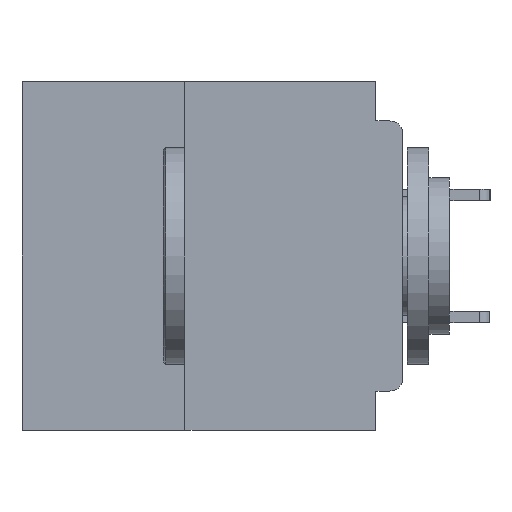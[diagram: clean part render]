
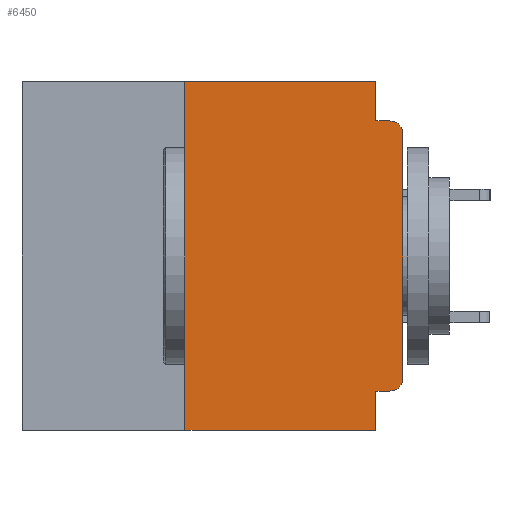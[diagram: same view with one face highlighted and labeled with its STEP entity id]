
A CAD part, left-side view. The second image highlights one B-rep face of the part: STEP entity #6450.
In plain terms, the highlighted planar face has unit normal (-1, 0, 0).
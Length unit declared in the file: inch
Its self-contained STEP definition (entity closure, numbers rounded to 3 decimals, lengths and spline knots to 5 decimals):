
#1854 = CARTESIAN_POINT ( 'NONE',  ( 0., 0.015, -0.34 ) ) ;
#1905 = LINE ( 'NONE', #18883, #39737 ) ;
#2397 = FACE_OUTER_BOUND ( 'NONE', #31106, .T. ) ;
#2887 = ORIENTED_EDGE ( 'NONE', *, *, #15777, .F. ) ;
#3714 = VERTEX_POINT ( 'NONE', #14060 ) ;
#4021 = CARTESIAN_POINT ( 'NONE',  ( 0., 0.25, -0.4 ) ) ;
#4457 = CARTESIAN_POINT ( 'NONE',  ( 0., 0., -0.34 ) ) ;
#5015 = CIRCLE ( 'NONE', #9411, 0.015 ) ;
#5131 = VERTEX_POINT ( 'NONE', #30509 ) ;
#5502 = EDGE_CURVE ( 'NONE', #15753, #28027, #8300, .T. ) ;
#5576 = DIRECTION ( 'NONE',  ( 0., 0., -1. ) ) ;
#5643 = ORIENTED_EDGE ( 'NONE', *, *, #18482, .F. ) ;
#5706 = DIRECTION ( 'NONE',  ( 0., -1., 0. ) ) ;
#5788 = CARTESIAN_POINT ( 'NONE',  ( 0., 0., 0. ) ) ;
#6450 = ADVANCED_FACE ( 'NONE', ( #2397 ), #8949, .F. ) ;
#6662 = DIRECTION ( 'NONE',  ( 0., -1., 0. ) ) ;
#6759 = CARTESIAN_POINT ( 'NONE',  ( 0., 0.031, -0.4 ) ) ;
#7590 = CARTESIAN_POINT ( 'NONE',  ( 0., 0.015, -0.06 ) ) ;
#8300 = LINE ( 'NONE', #6759, #27732 ) ;
#8949 = PLANE ( 'NONE',  #45016 ) ;
#9411 = AXIS2_PLACEMENT_3D ( 'NONE', #7590, #33226, #11280 ) ;
#10138 = LINE ( 'NONE', #44136, #16456 ) ;
#11251 = CARTESIAN_POINT ( 'NONE',  ( 0., 0.031, -0.355 ) ) ;
#11280 = DIRECTION ( 'NONE',  ( 0., 0., -1. ) ) ;
#13911 = LINE ( 'NONE', #4021, #22541 ) ;
#14024 = CARTESIAN_POINT ( 'NONE',  ( 0., 0.25, 0. ) ) ;
#14060 = CARTESIAN_POINT ( 'NONE',  ( 0., 0.015, -0.355 ) ) ;
#14962 = DIRECTION ( 'NONE',  ( 0., 0., 1. ) ) ;
#15753 = VERTEX_POINT ( 'NONE', #11251 ) ;
#15777 = EDGE_CURVE ( 'NONE', #5131, #25336, #13911, .T. ) ;
#16331 = DIRECTION ( 'NONE',  ( 0., 0., -1. ) ) ;
#16456 = VECTOR ( 'NONE', #18564, 39.37008 ) ;
#17638 = ORIENTED_EDGE ( 'NONE', *, *, #32061, .T. ) ;
#18025 = DIRECTION ( 'NONE',  ( 0., 0., -1. ) ) ;
#18482 = EDGE_CURVE ( 'NONE', #24933, #34365, #29122, .T. ) ;
#18564 = DIRECTION ( 'NONE',  ( 0., 1., 0. ) ) ;
#18883 = CARTESIAN_POINT ( 'NONE',  ( 0., 0.031, 0. ) ) ;
#19462 = VECTOR ( 'NONE', #6662, 39.37008 ) ;
#19937 = CARTESIAN_POINT ( 'NONE',  ( 0., 0.031, 0. ) ) ;
#20903 = VERTEX_POINT ( 'NONE', #39258 ) ;
#21000 = EDGE_CURVE ( 'NONE', #25336, #40945, #44535, .T. ) ;
#21565 = CARTESIAN_POINT ( 'NONE',  ( 0., 0.437, 0. ) ) ;
#22482 = ORIENTED_EDGE ( 'NONE', *, *, #45029, .T. ) ;
#22541 = VECTOR ( 'NONE', #14962, 39.37008 ) ;
#22747 = CARTESIAN_POINT ( 'NONE',  ( 0., 0.031, -0.045 ) ) ;
#23201 = ORIENTED_EDGE ( 'NONE', *, *, #30755, .T. ) ;
#24047 = AXIS2_PLACEMENT_3D ( 'NONE', #1854, #27508, #5576 ) ;
#24933 = VERTEX_POINT ( 'NONE', #22747 ) ;
#25336 = VERTEX_POINT ( 'NONE', #14024 ) ;
#25486 = EDGE_CURVE ( 'NONE', #20903, #34365, #5015, .T. ) ;
#26110 = VECTOR ( 'NONE', #5706, 39.37008 ) ;
#26769 = EDGE_CURVE ( 'NONE', #3714, #15753, #10138, .T. ) ;
#27401 = ORIENTED_EDGE ( 'NONE', *, *, #21000, .F. ) ;
#27508 = DIRECTION ( 'NONE',  ( -1., 0., 0. ) ) ;
#27618 = CARTESIAN_POINT ( 'NONE',  ( 0., 0.437, -0.4 ) ) ;
#27732 = VECTOR ( 'NONE', #18025, 39.37008 ) ;
#28027 = VERTEX_POINT ( 'NONE', #36148 ) ;
#28191 = EDGE_CURVE ( 'NONE', #40945, #24933, #1905, .T. ) ;
#29122 = LINE ( 'NONE', #46897, #19462 ) ;
#30314 = ORIENTED_EDGE ( 'NONE', *, *, #28191, .F. ) ;
#30509 = CARTESIAN_POINT ( 'NONE',  ( 0., 0.25, -0.4 ) ) ;
#30755 = EDGE_CURVE ( 'NONE', #3714, #33276, #33235, .T. ) ;
#31106 = EDGE_LOOP ( 'NONE', ( #17638, #46846, #5643, #30314, #27401, #2887, #22482, #43121, #33999, #23201 ) ) ;
#32061 = EDGE_CURVE ( 'NONE', #33276, #20903, #44654, .T. ) ;
#33226 = DIRECTION ( 'NONE',  ( -1., 0., 0. ) ) ;
#33235 = CIRCLE ( 'NONE', #24047, 0.015 ) ;
#33276 = VERTEX_POINT ( 'NONE', #4457 ) ;
#33999 = ORIENTED_EDGE ( 'NONE', *, *, #26769, .F. ) ;
#34365 = VERTEX_POINT ( 'NONE', #36075 ) ;
#34566 = CARTESIAN_POINT ( 'NONE',  ( 0., 0.437, 0. ) ) ;
#34895 = VECTOR ( 'NONE', #38755, 39.37008 ) ;
#36075 = CARTESIAN_POINT ( 'NONE',  ( 0., 0.015, -0.045 ) ) ;
#36148 = CARTESIAN_POINT ( 'NONE',  ( 0., 0.031, -0.4 ) ) ;
#38243 = DIRECTION ( 'NONE',  ( 1., 0., 0. ) ) ;
#38755 = DIRECTION ( 'NONE',  ( 0., 0., 1. ) ) ;
#39258 = CARTESIAN_POINT ( 'NONE',  ( 0., 0., -0.06 ) ) ;
#39737 = VECTOR ( 'NONE', #44470, 39.37008 ) ;
#39738 = DIRECTION ( 'NONE',  ( 0., -1., 0. ) ) ;
#40945 = VERTEX_POINT ( 'NONE', #19937 ) ;
#43121 = ORIENTED_EDGE ( 'NONE', *, *, #5502, .F. ) ;
#44136 = CARTESIAN_POINT ( 'NONE',  ( 0., 0., -0.355 ) ) ;
#44470 = DIRECTION ( 'NONE',  ( 0., 0., -1. ) ) ;
#44535 = LINE ( 'NONE', #21565, #45681 ) ;
#44654 = LINE ( 'NONE', #5788, #34895 ) ;
#45016 = AXIS2_PLACEMENT_3D ( 'NONE', #34566, #38243, #16331 ) ;
#45029 = EDGE_CURVE ( 'NONE', #5131, #28027, #45597, .T. ) ;
#45597 = LINE ( 'NONE', #27618, #26110 ) ;
#45681 = VECTOR ( 'NONE', #39738, 39.37008 ) ;
#46846 = ORIENTED_EDGE ( 'NONE', *, *, #25486, .T. ) ;
#46897 = CARTESIAN_POINT ( 'NONE',  ( 0., 0., -0.045 ) ) ;
